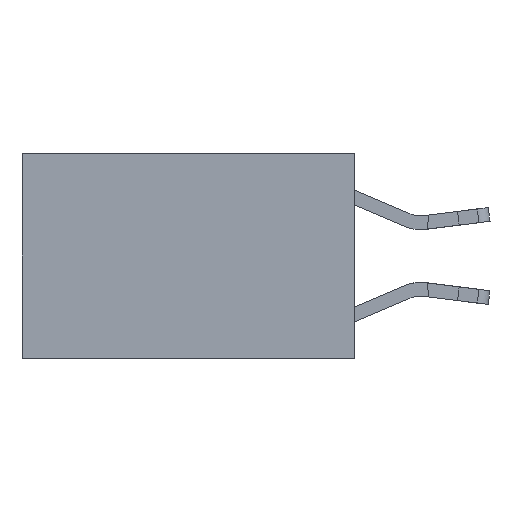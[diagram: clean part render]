
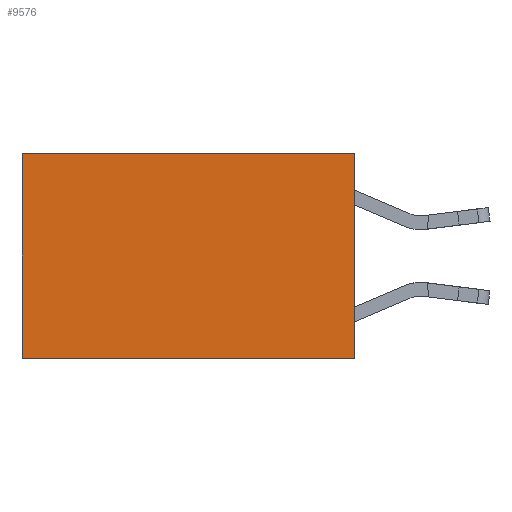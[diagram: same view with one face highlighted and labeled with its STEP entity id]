
A CAD part, left-side view. The second image highlights one B-rep face of the part: STEP entity #9576.
In plain terms, the highlighted planar face has unit normal (-1, 0, 0).
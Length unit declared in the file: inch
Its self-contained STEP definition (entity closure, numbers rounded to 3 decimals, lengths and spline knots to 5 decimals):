
#948 = VERTEX_POINT ( 'NONE', #9674 ) ;
#1068 = CARTESIAN_POINT ( 'NONE',  ( 0.2625, 0.6, 0. ) ) ;
#1119 = PLANE ( 'NONE',  #10664 ) ;
#1219 = CARTESIAN_POINT ( 'NONE',  ( 0.2625, 0., 0. ) ) ;
#1421 = ORIENTED_EDGE ( 'NONE', *, *, #6199, .T. ) ;
#1568 = EDGE_CURVE ( 'NONE', #3745, #948, #15015, .T. ) ;
#1615 = VECTOR ( 'NONE', #2349, 39.37008 ) ;
#2279 = VERTEX_POINT ( 'NONE', #10696 ) ;
#2287 = CARTESIAN_POINT ( 'NONE',  ( 0.2625, 0., -0.37 ) ) ;
#2349 = DIRECTION ( 'NONE',  ( 0., 0., -1. ) ) ;
#3745 = VERTEX_POINT ( 'NONE', #9073 ) ;
#3967 = DIRECTION ( 'NONE',  ( 1., 0., 0. ) ) ;
#5185 = DIRECTION ( 'NONE',  ( 0., 0., -1. ) ) ;
#5499 = EDGE_LOOP ( 'NONE', ( #1421, #7181, #8958, #15150 ) ) ;
#6095 = VECTOR ( 'NONE', #12315, 39.37008 ) ;
#6199 = EDGE_CURVE ( 'NONE', #2279, #948, #8590, .T. ) ;
#6284 = DIRECTION ( 'NONE',  ( 0., 1., 0. ) ) ;
#6580 = EDGE_CURVE ( 'NONE', #7308, #2279, #15760, .T. ) ;
#6966 = CARTESIAN_POINT ( 'NONE',  ( 0.2625, 0., 0. ) ) ;
#7181 = ORIENTED_EDGE ( 'NONE', *, *, #1568, .F. ) ;
#7308 = VERTEX_POINT ( 'NONE', #9097 ) ;
#7840 = VECTOR ( 'NONE', #9439, 39.37008 ) ;
#8590 = LINE ( 'NONE', #1068, #1615 ) ;
#8958 = ORIENTED_EDGE ( 'NONE', *, *, #14779, .F. ) ;
#9073 = CARTESIAN_POINT ( 'NONE',  ( 0.2625, 0., -0.37 ) ) ;
#9097 = CARTESIAN_POINT ( 'NONE',  ( 0.2625, 0., 0. ) ) ;
#9439 = DIRECTION ( 'NONE',  ( 0., 0., -1. ) ) ;
#9576 = ADVANCED_FACE ( 'NONE', ( #15012 ), #1119, .F. ) ;
#9674 = CARTESIAN_POINT ( 'NONE',  ( 0.2625, 0.6, -0.37 ) ) ;
#9747 = VECTOR ( 'NONE', #6284, 39.37008 ) ;
#10664 = AXIS2_PLACEMENT_3D ( 'NONE', #11400, #3967, #5185 ) ;
#10696 = CARTESIAN_POINT ( 'NONE',  ( 0.2625, 0.6, 0. ) ) ;
#11400 = CARTESIAN_POINT ( 'NONE',  ( 0.2625, 0., 0. ) ) ;
#12315 = DIRECTION ( 'NONE',  ( 0., 1., 0. ) ) ;
#13301 = LINE ( 'NONE', #6966, #7840 ) ;
#14779 = EDGE_CURVE ( 'NONE', #7308, #3745, #13301, .T. ) ;
#15012 = FACE_OUTER_BOUND ( 'NONE', #5499, .T. ) ;
#15015 = LINE ( 'NONE', #2287, #6095 ) ;
#15150 = ORIENTED_EDGE ( 'NONE', *, *, #6580, .T. ) ;
#15760 = LINE ( 'NONE', #1219, #9747 ) ;
